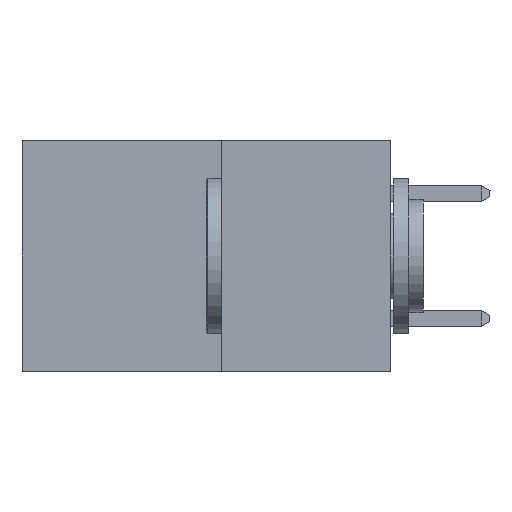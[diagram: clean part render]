
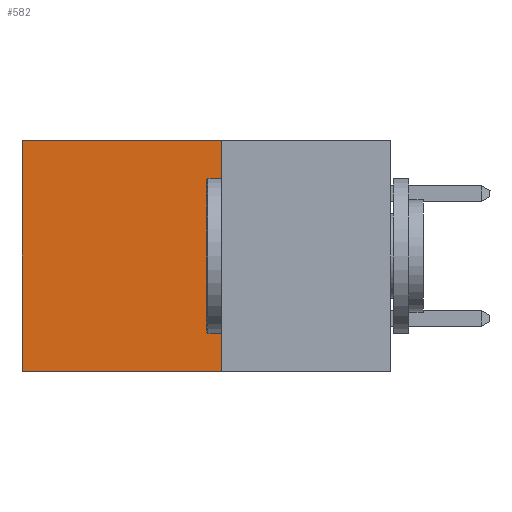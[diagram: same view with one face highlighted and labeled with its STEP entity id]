
A CAD part, left-side view. The second image highlights one B-rep face of the part: STEP entity #582.
In plain terms, the highlighted planar face has unit normal (-1, 0, 0).
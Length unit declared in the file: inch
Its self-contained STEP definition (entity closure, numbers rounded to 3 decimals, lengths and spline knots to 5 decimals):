
#582 = ADVANCED_FACE ( 'NONE', ( #17225 ), #11290, .F. ) ;
#596 = ORIENTED_EDGE ( 'NONE', *, *, #16777, .T. ) ;
#1392 = DIRECTION ( 'NONE',  ( 0., 0., -1. ) ) ;
#2452 = VERTEX_POINT ( 'NONE', #15169 ) ;
#2931 = CARTESIAN_POINT ( 'NONE',  ( 0.277, 0.27, 0. ) ) ;
#2973 = DIRECTION ( 'NONE',  ( 0., 1., 0. ) ) ;
#3291 = DIRECTION ( 'NONE',  ( 1., 0., 0. ) ) ;
#3478 = EDGE_CURVE ( 'NONE', #2452, #11149, #14487, .T. ) ;
#3496 = LINE ( 'NONE', #2931, #6904 ) ;
#3627 = EDGE_CURVE ( 'NONE', #17392, #6536, #3496, .T. ) ;
#4614 = LINE ( 'NONE', #18832, #15827 ) ;
#4635 = ORIENTED_EDGE ( 'NONE', *, *, #12590, .F. ) ;
#4921 = ORIENTED_EDGE ( 'NONE', *, *, #3478, .F. ) ;
#6536 = VERTEX_POINT ( 'NONE', #8201 ) ;
#6904 = VECTOR ( 'NONE', #2973, 39.37008 ) ;
#7145 = EDGE_LOOP ( 'NONE', ( #596, #4921, #4635, #15278 ) ) ;
#7327 = AXIS2_PLACEMENT_3D ( 'NONE', #17274, #3291, #13233 ) ;
#7542 = VECTOR ( 'NONE', #14888, 39.37008 ) ;
#8201 = CARTESIAN_POINT ( 'NONE',  ( 0.277, 0.59, 0. ) ) ;
#8501 = CARTESIAN_POINT ( 'NONE',  ( 0.277, 0.27, 0. ) ) ;
#9635 = VECTOR ( 'NONE', #15712, 39.37008 ) ;
#10962 = CARTESIAN_POINT ( 'NONE',  ( 0.277, 0.59, -0.37 ) ) ;
#11149 = VERTEX_POINT ( 'NONE', #10962 ) ;
#11290 = PLANE ( 'NONE',  #7327 ) ;
#12409 = LINE ( 'NONE', #13425, #7542 ) ;
#12590 = EDGE_CURVE ( 'NONE', #17392, #2452, #12409, .T. ) ;
#13233 = DIRECTION ( 'NONE',  ( 0., 0., -1. ) ) ;
#13425 = CARTESIAN_POINT ( 'NONE',  ( 0.277, 0.27, -0.37 ) ) ;
#14487 = LINE ( 'NONE', #15855, #9635 ) ;
#14888 = DIRECTION ( 'NONE',  ( 0., 0., -1. ) ) ;
#15169 = CARTESIAN_POINT ( 'NONE',  ( 0.277, 0.27, -0.37 ) ) ;
#15278 = ORIENTED_EDGE ( 'NONE', *, *, #3627, .T. ) ;
#15712 = DIRECTION ( 'NONE',  ( 0., 1., 0. ) ) ;
#15827 = VECTOR ( 'NONE', #1392, 39.37008 ) ;
#15855 = CARTESIAN_POINT ( 'NONE',  ( 0.277, 0.27, -0.37 ) ) ;
#16777 = EDGE_CURVE ( 'NONE', #6536, #11149, #4614, .T. ) ;
#17225 = FACE_OUTER_BOUND ( 'NONE', #7145, .T. ) ;
#17274 = CARTESIAN_POINT ( 'NONE',  ( 0.277, 0.27, -0.37 ) ) ;
#17392 = VERTEX_POINT ( 'NONE', #8501 ) ;
#18832 = CARTESIAN_POINT ( 'NONE',  ( 0.277, 0.59, -0.37 ) ) ;
